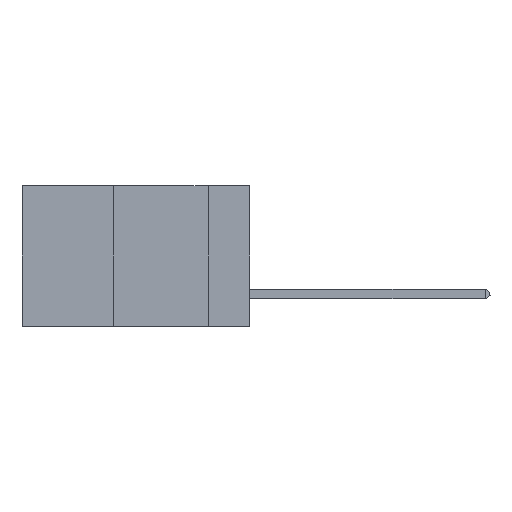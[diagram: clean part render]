
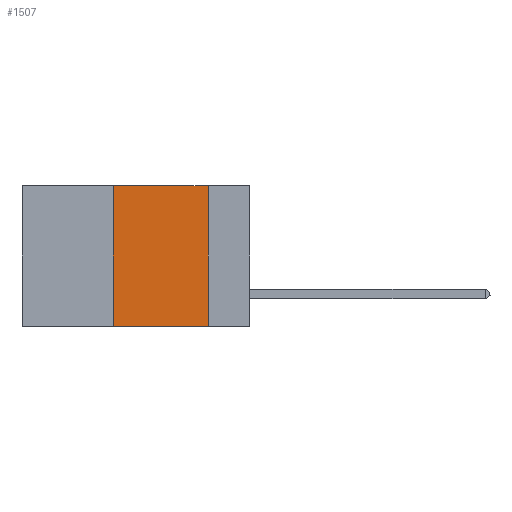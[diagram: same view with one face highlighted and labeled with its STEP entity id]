
A CAD part, left-side view. The second image highlights one B-rep face of the part: STEP entity #1507.
In plain terms, the highlighted planar face has unit normal (-1, 0, 0).
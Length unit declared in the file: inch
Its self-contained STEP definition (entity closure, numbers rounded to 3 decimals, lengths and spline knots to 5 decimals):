
#682 = DIRECTION ( 'NONE',  ( 0., 0., 1. ) ) ;
#713 = CARTESIAN_POINT ( 'NONE',  ( 0., 0.6, -0.37 ) ) ;
#718 = VERTEX_POINT ( 'NONE', #17100 ) ;
#1507 = ADVANCED_FACE ( 'NONE', ( #6556 ), #12011, .F. ) ;
#1511 = CARTESIAN_POINT ( 'NONE',  ( 0., 0.11, 0. ) ) ;
#2043 = DIRECTION ( 'NONE',  ( 0., 0., -1. ) ) ;
#2777 = LINE ( 'NONE', #9892, #7072 ) ;
#2879 = CARTESIAN_POINT ( 'NONE',  ( 0., 0.11, 0. ) ) ;
#3240 = AXIS2_PLACEMENT_3D ( 'NONE', #4285, #7300, #2043 ) ;
#3698 = EDGE_LOOP ( 'NONE', ( #7487, #14230, #15372, #11469 ) ) ;
#4285 = CARTESIAN_POINT ( 'NONE',  ( 0., 0.6, 0. ) ) ;
#5496 = CARTESIAN_POINT ( 'NONE',  ( 0., 0.36, -0.37 ) ) ;
#5727 = EDGE_CURVE ( 'NONE', #9266, #18694, #21572, .T. ) ;
#6209 = EDGE_CURVE ( 'NONE', #21022, #18694, #22129, .T. ) ;
#6277 = VECTOR ( 'NONE', #13352, 39.37008 ) ;
#6556 = FACE_OUTER_BOUND ( 'NONE', #3698, .T. ) ;
#7072 = VECTOR ( 'NONE', #682, 39.37008 ) ;
#7300 = DIRECTION ( 'NONE',  ( 1., 0., 0. ) ) ;
#7487 = ORIENTED_EDGE ( 'NONE', *, *, #6209, .F. ) ;
#9266 = VERTEX_POINT ( 'NONE', #5496 ) ;
#9892 = CARTESIAN_POINT ( 'NONE',  ( 0., 0.36, 0. ) ) ;
#11048 = VECTOR ( 'NONE', #19327, 39.37008 ) ;
#11469 = ORIENTED_EDGE ( 'NONE', *, *, #5727, .T. ) ;
#12011 = PLANE ( 'NONE',  #3240 ) ;
#13352 = DIRECTION ( 'NONE',  ( 0., -1., 0. ) ) ;
#14230 = ORIENTED_EDGE ( 'NONE', *, *, #19025, .F. ) ;
#15347 = DIRECTION ( 'NONE',  ( 0., -1., 0. ) ) ;
#15372 = ORIENTED_EDGE ( 'NONE', *, *, #19695, .F. ) ;
#16715 = VECTOR ( 'NONE', #15347, 39.37008 ) ;
#17100 = CARTESIAN_POINT ( 'NONE',  ( 0., 0.36, 0. ) ) ;
#18694 = VERTEX_POINT ( 'NONE', #23470 ) ;
#19025 = EDGE_CURVE ( 'NONE', #718, #21022, #20573, .T. ) ;
#19327 = DIRECTION ( 'NONE',  ( 0., 0., -1. ) ) ;
#19695 = EDGE_CURVE ( 'NONE', #9266, #718, #2777, .T. ) ;
#20573 = LINE ( 'NONE', #22337, #6277 ) ;
#21022 = VERTEX_POINT ( 'NONE', #1511 ) ;
#21572 = LINE ( 'NONE', #713, #16715 ) ;
#22129 = LINE ( 'NONE', #2879, #11048 ) ;
#22337 = CARTESIAN_POINT ( 'NONE',  ( 0., 0.6, 0. ) ) ;
#23470 = CARTESIAN_POINT ( 'NONE',  ( 0., 0.11, -0.37 ) ) ;
